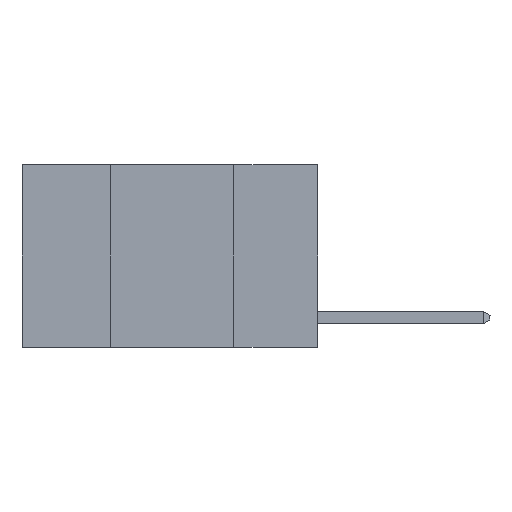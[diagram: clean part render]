
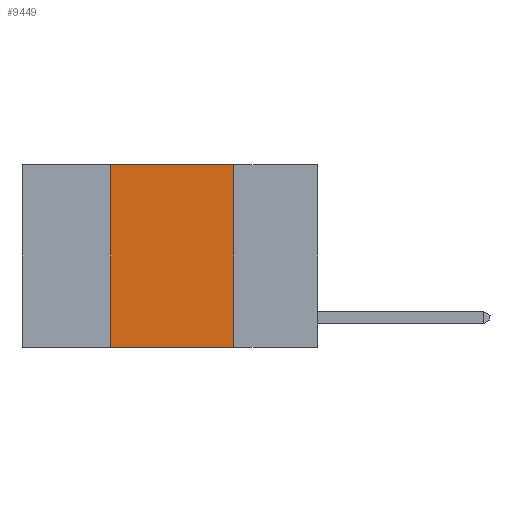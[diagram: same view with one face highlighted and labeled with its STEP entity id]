
A CAD part, left-side view. The second image highlights one B-rep face of the part: STEP entity #9449.
In plain terms, the highlighted planar face has unit normal (-1, 0, 0).
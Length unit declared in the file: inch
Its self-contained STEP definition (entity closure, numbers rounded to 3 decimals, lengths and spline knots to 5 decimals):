
#291 = EDGE_LOOP ( 'NONE', ( #8474, #2852, #10800, #17630 ) ) ;
#408 = EDGE_CURVE ( 'NONE', #8404, #2468, #5691, .T. ) ;
#1166 = AXIS2_PLACEMENT_3D ( 'NONE', #3743, #13614, #14979 ) ;
#1238 = CARTESIAN_POINT ( 'NONE',  ( 0., 0.42, 0. ) ) ;
#1747 = VERTEX_POINT ( 'NONE', #8279 ) ;
#2468 = VERTEX_POINT ( 'NONE', #5317 ) ;
#2623 = VECTOR ( 'NONE', #6510, 39.37008 ) ;
#2852 = ORIENTED_EDGE ( 'NONE', *, *, #408, .F. ) ;
#3409 = EDGE_CURVE ( 'NONE', #2468, #9324, #9439, .T. ) ;
#3587 = LINE ( 'NONE', #1238, #2623 ) ;
#3743 = CARTESIAN_POINT ( 'NONE',  ( 0., 0.6, 0. ) ) ;
#4539 = VECTOR ( 'NONE', #15766, 39.37008 ) ;
#4965 = VECTOR ( 'NONE', #14970, 39.37008 ) ;
#5317 = CARTESIAN_POINT ( 'NONE',  ( 0., 0.17, 0. ) ) ;
#5691 = LINE ( 'NONE', #14278, #4539 ) ;
#6510 = DIRECTION ( 'NONE',  ( 0., 0., 1. ) ) ;
#6769 = EDGE_CURVE ( 'NONE', #1747, #9324, #9970, .T. ) ;
#8004 = FACE_OUTER_BOUND ( 'NONE', #291, .T. ) ;
#8279 = CARTESIAN_POINT ( 'NONE',  ( 0., 0.42, -0.37 ) ) ;
#8404 = VERTEX_POINT ( 'NONE', #11837 ) ;
#8474 = ORIENTED_EDGE ( 'NONE', *, *, #3409, .F. ) ;
#9324 = VERTEX_POINT ( 'NONE', #17275 ) ;
#9439 = LINE ( 'NONE', #12258, #4965 ) ;
#9449 = ADVANCED_FACE ( 'NONE', ( #8004 ), #16276, .F. ) ;
#9970 = LINE ( 'NONE', #16373, #10347 ) ;
#10347 = VECTOR ( 'NONE', #17900, 39.37008 ) ;
#10800 = ORIENTED_EDGE ( 'NONE', *, *, #11983, .F. ) ;
#11837 = CARTESIAN_POINT ( 'NONE',  ( 0., 0.42, 0. ) ) ;
#11983 = EDGE_CURVE ( 'NONE', #1747, #8404, #3587, .T. ) ;
#12258 = CARTESIAN_POINT ( 'NONE',  ( 0., 0.17, 0. ) ) ;
#13614 = DIRECTION ( 'NONE',  ( 1., 0., 0. ) ) ;
#14278 = CARTESIAN_POINT ( 'NONE',  ( 0., 0.6, 0. ) ) ;
#14970 = DIRECTION ( 'NONE',  ( 0., 0., -1. ) ) ;
#14979 = DIRECTION ( 'NONE',  ( 0., 0., -1. ) ) ;
#15766 = DIRECTION ( 'NONE',  ( 0., -1., 0. ) ) ;
#16276 = PLANE ( 'NONE',  #1166 ) ;
#16373 = CARTESIAN_POINT ( 'NONE',  ( 0., 0.6, -0.37 ) ) ;
#17275 = CARTESIAN_POINT ( 'NONE',  ( 0., 0.17, -0.37 ) ) ;
#17630 = ORIENTED_EDGE ( 'NONE', *, *, #6769, .T. ) ;
#17900 = DIRECTION ( 'NONE',  ( 0., -1., 0. ) ) ;
